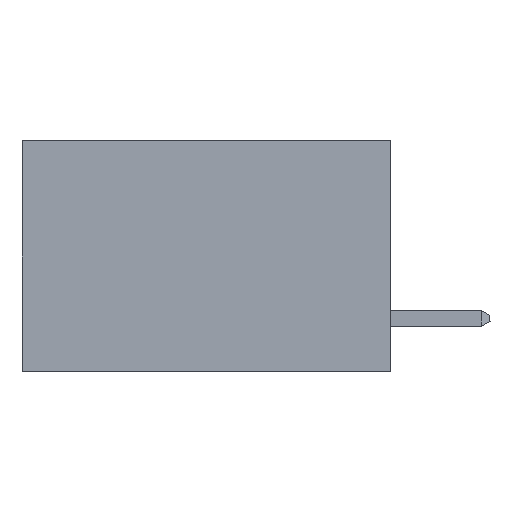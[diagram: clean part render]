
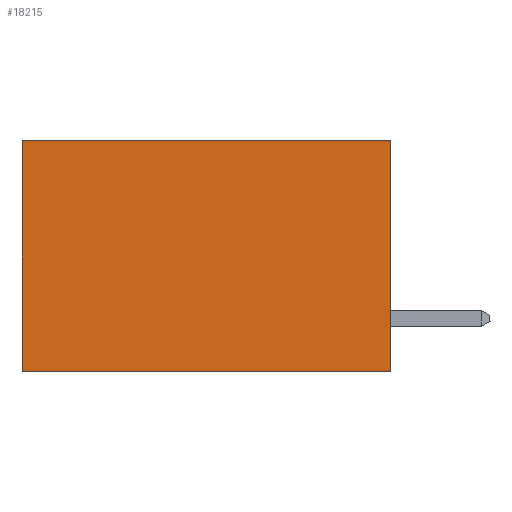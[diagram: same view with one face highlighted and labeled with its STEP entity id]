
A CAD part, left-side view. The second image highlights one B-rep face of the part: STEP entity #18215.
In plain terms, the highlighted planar face has unit normal (-1, 0, 0).
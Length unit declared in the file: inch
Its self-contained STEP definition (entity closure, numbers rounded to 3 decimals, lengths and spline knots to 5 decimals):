
#109 = LINE ( 'NONE', #14532, #679 ) ;
#177 = VERTEX_POINT ( 'NONE', #20086 ) ;
#440 = EDGE_LOOP ( 'NONE', ( #6184, #14218, #11747, #6088 ) ) ;
#679 = VECTOR ( 'NONE', #3792, 39.37008 ) ;
#1758 = VERTEX_POINT ( 'NONE', #18351 ) ;
#2075 = EDGE_CURVE ( 'NONE', #14833, #177, #2082, .T. ) ;
#2082 = LINE ( 'NONE', #7012, #11704 ) ;
#3792 = DIRECTION ( 'NONE',  ( 0., 0., -1. ) ) ;
#4493 = PLANE ( 'NONE',  #5476 ) ;
#5476 = AXIS2_PLACEMENT_3D ( 'NONE', #16931, #18684, #8112 ) ;
#6088 = ORIENTED_EDGE ( 'NONE', *, *, #21360, .T. ) ;
#6184 = ORIENTED_EDGE ( 'NONE', *, *, #9481, .T. ) ;
#6608 = FACE_OUTER_BOUND ( 'NONE', #440, .T. ) ;
#7012 = CARTESIAN_POINT ( 'NONE',  ( 0.277, 0., -0.37 ) ) ;
#7627 = CARTESIAN_POINT ( 'NONE',  ( 0.277, 0., 0. ) ) ;
#8112 = DIRECTION ( 'NONE',  ( 0., 0., -1. ) ) ;
#9481 = EDGE_CURVE ( 'NONE', #1758, #177, #13110, .T. ) ;
#10575 = DIRECTION ( 'NONE',  ( 0., 1., 0. ) ) ;
#11085 = CARTESIAN_POINT ( 'NONE',  ( 0.277, 0., -0.37 ) ) ;
#11704 = VECTOR ( 'NONE', #13563, 39.37008 ) ;
#11747 = ORIENTED_EDGE ( 'NONE', *, *, #19786, .F. ) ;
#13110 = LINE ( 'NONE', #14751, #17188 ) ;
#13563 = DIRECTION ( 'NONE',  ( 0., 1., 0. ) ) ;
#14066 = CARTESIAN_POINT ( 'NONE',  ( 0.277, 0., 0. ) ) ;
#14218 = ORIENTED_EDGE ( 'NONE', *, *, #2075, .F. ) ;
#14532 = CARTESIAN_POINT ( 'NONE',  ( 0.277, 0., -0.37 ) ) ;
#14730 = DIRECTION ( 'NONE',  ( 0., 0., -1. ) ) ;
#14751 = CARTESIAN_POINT ( 'NONE',  ( 0.277, 0.59, -0.37 ) ) ;
#14833 = VERTEX_POINT ( 'NONE', #11085 ) ;
#16034 = VERTEX_POINT ( 'NONE', #7627 ) ;
#16931 = CARTESIAN_POINT ( 'NONE',  ( 0.277, 0., -0.37 ) ) ;
#17188 = VECTOR ( 'NONE', #14730, 39.37008 ) ;
#18215 = ADVANCED_FACE ( 'NONE', ( #6608 ), #4493, .F. ) ;
#18351 = CARTESIAN_POINT ( 'NONE',  ( 0.277, 0.59, 0. ) ) ;
#18684 = DIRECTION ( 'NONE',  ( 1., 0., 0. ) ) ;
#19786 = EDGE_CURVE ( 'NONE', #16034, #14833, #109, .T. ) ;
#20086 = CARTESIAN_POINT ( 'NONE',  ( 0.277, 0.59, -0.37 ) ) ;
#20379 = VECTOR ( 'NONE', #10575, 39.37008 ) ;
#20913 = LINE ( 'NONE', #14066, #20379 ) ;
#21360 = EDGE_CURVE ( 'NONE', #16034, #1758, #20913, .T. ) ;
